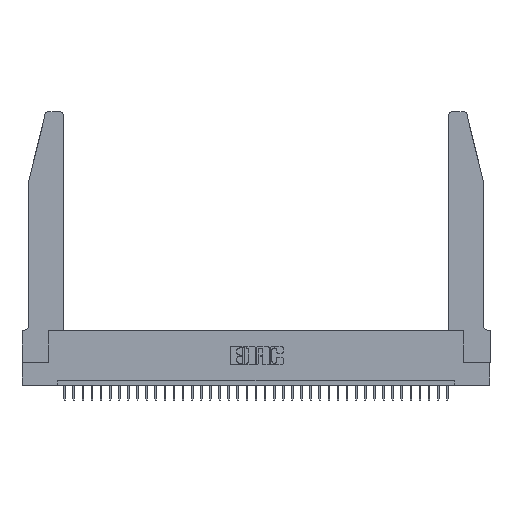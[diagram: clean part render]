
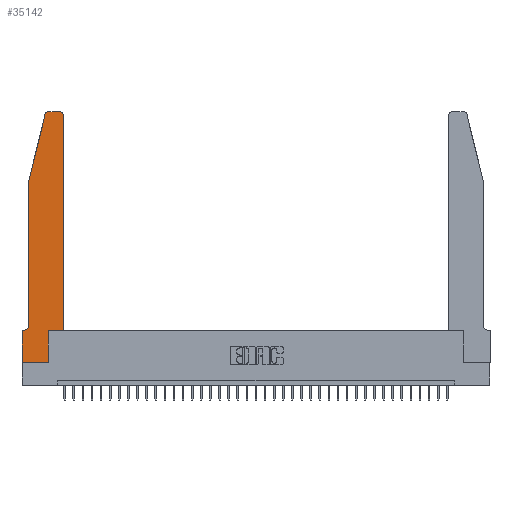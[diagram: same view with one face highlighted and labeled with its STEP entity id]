
A CAD part, top view. The second image highlights one B-rep face of the part: STEP entity #35142.
In plain terms, the highlighted planar face has unit normal (0, 0, 1).
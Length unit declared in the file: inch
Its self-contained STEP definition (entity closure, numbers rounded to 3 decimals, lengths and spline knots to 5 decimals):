
#176 = EDGE_CURVE ( 'NONE', #22323, #16999, #35525, .T. ) ;
#225 = DIRECTION ( 'NONE',  ( 1., 0., 0. ) ) ;
#896 = CARTESIAN_POINT ( 'NONE',  ( 0.4505, 0.35, 0.37 ) ) ;
#1460 = LINE ( 'NONE', #18081, #22429 ) ;
#1648 = CARTESIAN_POINT ( 'NONE',  ( 0.284, 2.75, 0.37 ) ) ;
#1732 = EDGE_CURVE ( 'NONE', #26270, #10427, #1460, .T. ) ;
#2010 = CARTESIAN_POINT ( 'NONE',  ( 0.4205, 2.72, 0.37 ) ) ;
#2635 = LINE ( 'NONE', #8951, #15115 ) ;
#3442 = CARTESIAN_POINT ( 'NONE',  ( 0.0055, 0.35, 0.37 ) ) ;
#5158 = VECTOR ( 'NONE', #18187, 39.37008 ) ;
#5481 = VECTOR ( 'NONE', #14184, 39.37008 ) ;
#5669 = ORIENTED_EDGE ( 'NONE', *, *, #7916, .T. ) ;
#5876 = LINE ( 'NONE', #896, #17953 ) ;
#6023 = CARTESIAN_POINT ( 'NONE',  ( 0.25487, 2.72718, 0.37 ) ) ;
#6692 = CARTESIAN_POINT ( 'NONE',  ( 0.4505, 0.35, 0.37 ) ) ;
#6734 = DIRECTION ( 'NONE',  ( 0., -1., 0. ) ) ;
#6740 = ORIENTED_EDGE ( 'NONE', *, *, #23952, .T. ) ;
#7135 = DIRECTION ( 'NONE',  ( -0.239, -0.971, 0. ) ) ;
#7916 = EDGE_CURVE ( 'NONE', #10427, #22323, #17707, .T. ) ;
#7921 = ORIENTED_EDGE ( 'NONE', *, *, #13804, .T. ) ;
#7950 = CARTESIAN_POINT ( 'NONE',  ( 0.0755, 0.35, 0.37 ) ) ;
#8343 = CARTESIAN_POINT ( 'NONE',  ( 0.2865, 0.35, 0.37 ) ) ;
#8457 = CARTESIAN_POINT ( 'NONE',  ( 0., 0.35, 0.37 ) ) ;
#8867 = VERTEX_POINT ( 'NONE', #1648 ) ;
#8887 = PLANE ( 'NONE',  #11910 ) ;
#8951 = CARTESIAN_POINT ( 'NONE',  ( 0.2865, 0.35, 0.37 ) ) ;
#8978 = CARTESIAN_POINT ( 'NONE',  ( 0.0755, 2., 0.37 ) ) ;
#9332 = CARTESIAN_POINT ( 'NONE',  ( 0., 0., 0.37 ) ) ;
#9534 = CARTESIAN_POINT ( 'NONE',  ( 0.4505, 0.35, 0.37 ) ) ;
#9703 = VERTEX_POINT ( 'NONE', #21043 ) ;
#10427 = VERTEX_POINT ( 'NONE', #27058 ) ;
#11910 = AXIS2_PLACEMENT_3D ( 'NONE', #14494, #14978, #225 ) ;
#12003 = EDGE_CURVE ( 'NONE', #36267, #14138, #30419, .T. ) ;
#13582 = CARTESIAN_POINT ( 'NONE',  ( 0.0055, 0.42, 0.37 ) ) ;
#13804 = EDGE_CURVE ( 'NONE', #35161, #26270, #27578, .T. ) ;
#13880 = ORIENTED_EDGE ( 'NONE', *, *, #20266, .T. ) ;
#13927 = VECTOR ( 'NONE', #14432, 39.37008 ) ;
#14138 = VERTEX_POINT ( 'NONE', #9534 ) ;
#14184 = DIRECTION ( 'NONE',  ( 1., 0., 0. ) ) ;
#14250 = EDGE_LOOP ( 'NONE', ( #26301, #14301, #7921, #28684, #5669, #28246, #13880, #15045, #33083, #24429, #15078, #6740 ) ) ;
#14253 = DIRECTION ( 'NONE',  ( 1., 0., 0. ) ) ;
#14301 = ORIENTED_EDGE ( 'NONE', *, *, #19050, .T. ) ;
#14432 = DIRECTION ( 'NONE',  ( -1., 0., 0. ) ) ;
#14494 = CARTESIAN_POINT ( 'NONE',  ( 0., 0.35, 0.37 ) ) ;
#14978 = DIRECTION ( 'NONE',  ( 0., 0., 1. ) ) ;
#14985 = DIRECTION ( 'NONE',  ( 0., 1., 0. ) ) ;
#15045 = ORIENTED_EDGE ( 'NONE', *, *, #33272, .T. ) ;
#15078 = ORIENTED_EDGE ( 'NONE', *, *, #21948, .T. ) ;
#15115 = VECTOR ( 'NONE', #26553, 39.37008 ) ;
#16376 = VERTEX_POINT ( 'NONE', #24368 ) ;
#16999 = VERTEX_POINT ( 'NONE', #8457 ) ;
#17707 = CIRCLE ( 'NONE', #31650, 0.07 ) ;
#17953 = VECTOR ( 'NONE', #14985, 39.37008 ) ;
#18081 = CARTESIAN_POINT ( 'NONE',  ( 0.0755, 2., 0.37 ) ) ;
#18187 = DIRECTION ( 'NONE',  ( 0., -1., 0. ) ) ;
#18900 = LINE ( 'NONE', #36462, #5481 ) ;
#19050 = EDGE_CURVE ( 'NONE', #8867, #35161, #20013, .T. ) ;
#19321 = DIRECTION ( 'NONE',  ( -1., 0., 0. ) ) ;
#20013 = CIRCLE ( 'NONE', #22293, 0.03 ) ;
#20020 = CIRCLE ( 'NONE', #21695, 0.03 ) ;
#20266 = EDGE_CURVE ( 'NONE', #16999, #32995, #33323, .T. ) ;
#20387 = CARTESIAN_POINT ( 'NONE',  ( 0., 0., 0.37 ) ) ;
#21043 = CARTESIAN_POINT ( 'NONE',  ( 0.4205, 2.75, 0.37 ) ) ;
#21540 = VERTEX_POINT ( 'NONE', #31095 ) ;
#21645 = VECTOR ( 'NONE', #28625, 39.37008 ) ;
#21695 = AXIS2_PLACEMENT_3D ( 'NONE', #2010, #30712, #21972 ) ;
#21948 = EDGE_CURVE ( 'NONE', #14138, #21540, #5876, .T. ) ;
#21972 = DIRECTION ( 'NONE',  ( 1., 0., 0. ) ) ;
#22293 = AXIS2_PLACEMENT_3D ( 'NONE', #37030, #31366, #14253 ) ;
#22296 = EDGE_CURVE ( 'NONE', #9703, #8867, #31333, .T. ) ;
#22323 = VERTEX_POINT ( 'NONE', #3442 ) ;
#22429 = VECTOR ( 'NONE', #6734, 39.37008 ) ;
#23516 = EDGE_CURVE ( 'NONE', #16376, #36267, #2635, .T. ) ;
#23952 = EDGE_CURVE ( 'NONE', #21540, #9703, #20020, .T. ) ;
#23972 = VECTOR ( 'NONE', #7135, 39.37008 ) ;
#24368 = CARTESIAN_POINT ( 'NONE',  ( 0.2865, 0., 0.37 ) ) ;
#24429 = ORIENTED_EDGE ( 'NONE', *, *, #12003, .T. ) ;
#24521 = FACE_OUTER_BOUND ( 'NONE', #14250, .T. ) ;
#26270 = VERTEX_POINT ( 'NONE', #8978 ) ;
#26301 = ORIENTED_EDGE ( 'NONE', *, *, #22296, .T. ) ;
#26553 = DIRECTION ( 'NONE',  ( 0., 1., 0. ) ) ;
#27058 = CARTESIAN_POINT ( 'NONE',  ( 0.0755, 0.42, 0.37 ) ) ;
#27578 = LINE ( 'NONE', #30090, #23972 ) ;
#28246 = ORIENTED_EDGE ( 'NONE', *, *, #176, .T. ) ;
#28625 = DIRECTION ( 'NONE',  ( -1., 0., 0. ) ) ;
#28684 = ORIENTED_EDGE ( 'NONE', *, *, #1732, .T. ) ;
#29077 = CARTESIAN_POINT ( 'NONE',  ( 0.2605, 2.75, 0.37 ) ) ;
#30090 = CARTESIAN_POINT ( 'NONE',  ( 0.0755, 2., 0.37 ) ) ;
#30419 = LINE ( 'NONE', #6692, #32169 ) ;
#30712 = DIRECTION ( 'NONE',  ( 0., 0., 1. ) ) ;
#31095 = CARTESIAN_POINT ( 'NONE',  ( 0.4505, 2.72, 0.37 ) ) ;
#31333 = LINE ( 'NONE', #29077, #13927 ) ;
#31366 = DIRECTION ( 'NONE',  ( 0., 0., 1. ) ) ;
#31650 = AXIS2_PLACEMENT_3D ( 'NONE', #13582, #33568, #19321 ) ;
#32169 = VECTOR ( 'NONE', #35934, 39.37008 ) ;
#32995 = VERTEX_POINT ( 'NONE', #20387 ) ;
#33083 = ORIENTED_EDGE ( 'NONE', *, *, #23516, .T. ) ;
#33272 = EDGE_CURVE ( 'NONE', #32995, #16376, #18900, .T. ) ;
#33323 = LINE ( 'NONE', #9332, #5158 ) ;
#33568 = DIRECTION ( 'NONE',  ( 0., 0., -1. ) ) ;
#35142 = ADVANCED_FACE ( 'NONE', ( #24521 ), #8887, .T. ) ;
#35161 = VERTEX_POINT ( 'NONE', #6023 ) ;
#35525 = LINE ( 'NONE', #7950, #21645 ) ;
#35934 = DIRECTION ( 'NONE',  ( 1., 0., 0. ) ) ;
#36267 = VERTEX_POINT ( 'NONE', #8343 ) ;
#36462 = CARTESIAN_POINT ( 'NONE',  ( 0., 0., 0.37 ) ) ;
#37030 = CARTESIAN_POINT ( 'NONE',  ( 0.284, 2.72, 0.37 ) ) ;
